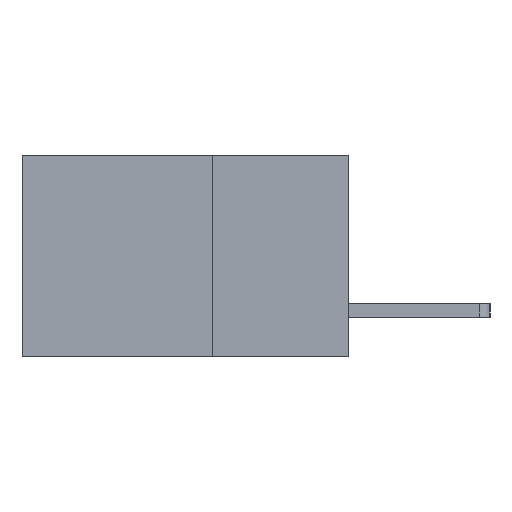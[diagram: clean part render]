
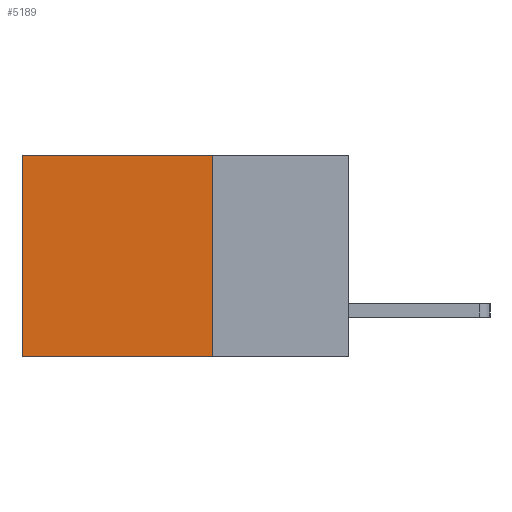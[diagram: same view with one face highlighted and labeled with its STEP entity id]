
A CAD part, left-side view. The second image highlights one B-rep face of the part: STEP entity #5189.
In plain terms, the highlighted planar face has unit normal (-1, 0, 0).
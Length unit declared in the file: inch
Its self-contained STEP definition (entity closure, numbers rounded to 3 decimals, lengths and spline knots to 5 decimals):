
#309 = LINE ( 'NONE', #5468, #8291 ) ;
#587 = ORIENTED_EDGE ( 'NONE', *, *, #9928, .T. ) ;
#1589 = AXIS2_PLACEMENT_3D ( 'NONE', #6838, #6829, #6827 ) ;
#2017 = VECTOR ( 'NONE', #9339, 39.37008 ) ;
#2103 = VERTEX_POINT ( 'NONE', #6595 ) ;
#2265 = LINE ( 'NONE', #8595, #2017 ) ;
#2466 = DIRECTION ( 'NONE',  ( 0., 0., -1. ) ) ;
#3518 = EDGE_LOOP ( 'NONE', ( #587, #7727, #8472, #5526 ) ) ;
#4414 = VERTEX_POINT ( 'NONE', #9688 ) ;
#4593 = EDGE_CURVE ( 'NONE', #6950, #4414, #9691, .T. ) ;
#5189 = ADVANCED_FACE ( 'NONE', ( #8298 ), #6872, .F. ) ;
#5388 = DIRECTION ( 'NONE',  ( 0., 0., -1. ) ) ;
#5468 = CARTESIAN_POINT ( 'NONE',  ( 0.2615, 0.25, -0.37 ) ) ;
#5526 = ORIENTED_EDGE ( 'NONE', *, *, #7833, .T. ) ;
#5639 = EDGE_CURVE ( 'NONE', #8702, #6950, #309, .T. ) ;
#5657 = LINE ( 'NONE', #7815, #6131 ) ;
#5676 = VECTOR ( 'NONE', #8932, 39.37008 ) ;
#6131 = VECTOR ( 'NONE', #2466, 39.37008 ) ;
#6595 = CARTESIAN_POINT ( 'NONE',  ( 0.2615, 0.6, 0. ) ) ;
#6827 = DIRECTION ( 'NONE',  ( 0., 0., -1. ) ) ;
#6829 = DIRECTION ( 'NONE',  ( 1., 0., 0. ) ) ;
#6838 = CARTESIAN_POINT ( 'NONE',  ( 0.2615, 0.25, -0.37 ) ) ;
#6872 = PLANE ( 'NONE',  #1589 ) ;
#6950 = VERTEX_POINT ( 'NONE', #7537 ) ;
#7537 = CARTESIAN_POINT ( 'NONE',  ( 0.2615, 0.25, -0.37 ) ) ;
#7727 = ORIENTED_EDGE ( 'NONE', *, *, #4593, .F. ) ;
#7815 = CARTESIAN_POINT ( 'NONE',  ( 0.2615, 0.6, -0.37 ) ) ;
#7833 = EDGE_CURVE ( 'NONE', #8702, #2103, #2265, .T. ) ;
#8291 = VECTOR ( 'NONE', #5388, 39.37008 ) ;
#8298 = FACE_OUTER_BOUND ( 'NONE', #3518, .T. ) ;
#8472 = ORIENTED_EDGE ( 'NONE', *, *, #5639, .F. ) ;
#8595 = CARTESIAN_POINT ( 'NONE',  ( 0.2615, 0.25, 0. ) ) ;
#8702 = VERTEX_POINT ( 'NONE', #9705 ) ;
#8923 = CARTESIAN_POINT ( 'NONE',  ( 0.2615, 0.25, -0.37 ) ) ;
#8932 = DIRECTION ( 'NONE',  ( 0., 1., 0. ) ) ;
#9339 = DIRECTION ( 'NONE',  ( 0., 1., 0. ) ) ;
#9688 = CARTESIAN_POINT ( 'NONE',  ( 0.2615, 0.6, -0.37 ) ) ;
#9691 = LINE ( 'NONE', #8923, #5676 ) ;
#9705 = CARTESIAN_POINT ( 'NONE',  ( 0.2615, 0.25, 0. ) ) ;
#9928 = EDGE_CURVE ( 'NONE', #2103, #4414, #5657, .T. ) ;
